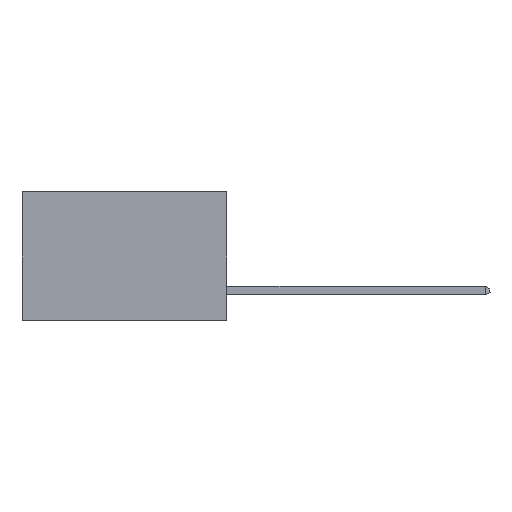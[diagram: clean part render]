
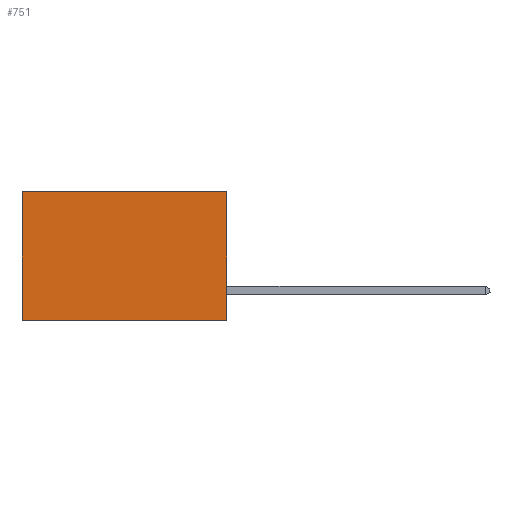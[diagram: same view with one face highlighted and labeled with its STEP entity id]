
A CAD part, left-side view. The second image highlights one B-rep face of the part: STEP entity #751.
In plain terms, the highlighted planar face has unit normal (-1, 0, 0).
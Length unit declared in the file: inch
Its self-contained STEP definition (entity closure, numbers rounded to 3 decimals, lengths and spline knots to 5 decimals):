
#468 = LINE ( 'NONE', #12214, #23532 ) ;
#751 = ADVANCED_FACE ( 'NONE', ( #1213 ), #9713, .F. ) ;
#1078 = EDGE_CURVE ( 'NONE', #8242, #5791, #468, .T. ) ;
#1211 = LINE ( 'NONE', #18940, #18898 ) ;
#1213 = FACE_OUTER_BOUND ( 'NONE', #27017, .T. ) ;
#1460 = EDGE_CURVE ( 'NONE', #6026, #5791, #1211, .T. ) ;
#1871 = EDGE_CURVE ( 'NONE', #5829, #8242, #8023, .T. ) ;
#4931 = VECTOR ( 'NONE', #19610, 39.37008 ) ;
#5122 = CARTESIAN_POINT ( 'NONE',  ( 0.277, 0., 0. ) ) ;
#5791 = VERTEX_POINT ( 'NONE', #6679 ) ;
#5829 = VERTEX_POINT ( 'NONE', #5122 ) ;
#6026 = VERTEX_POINT ( 'NONE', #23168 ) ;
#6679 = CARTESIAN_POINT ( 'NONE',  ( 0.277, 0.59, -0.37 ) ) ;
#7945 = AXIS2_PLACEMENT_3D ( 'NONE', #11735, #10287, #22670 ) ;
#8023 = LINE ( 'NONE', #8038, #19595 ) ;
#8038 = CARTESIAN_POINT ( 'NONE',  ( 0.277, 0., 0. ) ) ;
#8242 = VERTEX_POINT ( 'NONE', #19842 ) ;
#9713 = PLANE ( 'NONE',  #7945 ) ;
#10217 = DIRECTION ( 'NONE',  ( 0., 1., 0. ) ) ;
#10287 = DIRECTION ( 'NONE',  ( 1., 0., 0. ) ) ;
#11735 = CARTESIAN_POINT ( 'NONE',  ( 0.277, 0., -0.37 ) ) ;
#11906 = ORIENTED_EDGE ( 'NONE', *, *, #1460, .F. ) ;
#12214 = CARTESIAN_POINT ( 'NONE',  ( 0.277, 0.59, -0.37 ) ) ;
#16021 = ORIENTED_EDGE ( 'NONE', *, *, #1078, .T. ) ;
#16714 = ORIENTED_EDGE ( 'NONE', *, *, #1871, .T. ) ;
#17187 = LINE ( 'NONE', #17319, #4931 ) ;
#17319 = CARTESIAN_POINT ( 'NONE',  ( 0.277, 0., -0.37 ) ) ;
#18898 = VECTOR ( 'NONE', #10217, 39.37008 ) ;
#18940 = CARTESIAN_POINT ( 'NONE',  ( 0.277, 0., -0.37 ) ) ;
#19595 = VECTOR ( 'NONE', #28955, 39.37008 ) ;
#19610 = DIRECTION ( 'NONE',  ( 0., 0., -1. ) ) ;
#19842 = CARTESIAN_POINT ( 'NONE',  ( 0.277, 0.59, 0. ) ) ;
#22670 = DIRECTION ( 'NONE',  ( 0., 0., -1. ) ) ;
#23168 = CARTESIAN_POINT ( 'NONE',  ( 0.277, 0., -0.37 ) ) ;
#23532 = VECTOR ( 'NONE', #26664, 39.37008 ) ;
#24694 = ORIENTED_EDGE ( 'NONE', *, *, #26620, .F. ) ;
#26620 = EDGE_CURVE ( 'NONE', #5829, #6026, #17187, .T. ) ;
#26664 = DIRECTION ( 'NONE',  ( 0., 0., -1. ) ) ;
#27017 = EDGE_LOOP ( 'NONE', ( #16021, #11906, #24694, #16714 ) ) ;
#28955 = DIRECTION ( 'NONE',  ( 0., 1., 0. ) ) ;
